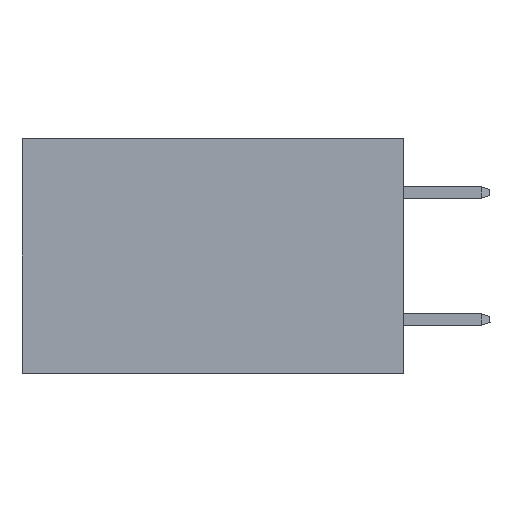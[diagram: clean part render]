
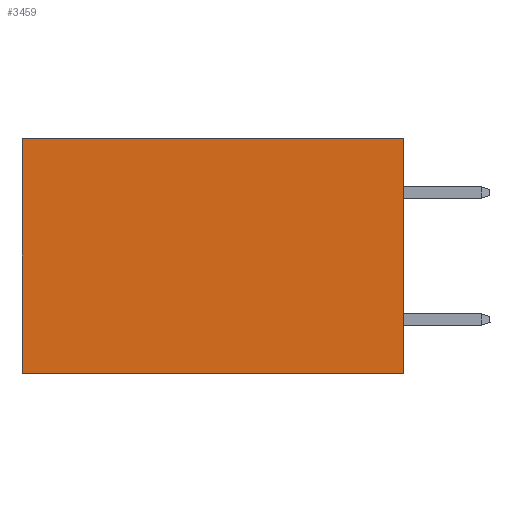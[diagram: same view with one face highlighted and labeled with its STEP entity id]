
A CAD part, left-side view. The second image highlights one B-rep face of the part: STEP entity #3459.
In plain terms, the highlighted planar face has unit normal (-1, 0, 0).
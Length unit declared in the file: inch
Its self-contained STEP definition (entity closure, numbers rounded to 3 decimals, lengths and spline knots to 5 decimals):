
#1199 = VERTEX_POINT ( 'NONE', #18235 ) ;
#1871 = DIRECTION ( 'NONE',  ( 0., 0., -1. ) ) ;
#3299 = DIRECTION ( 'NONE',  ( 1., 0., 0. ) ) ;
#3459 = ADVANCED_FACE ( 'NONE', ( #24115 ), #23495, .F. ) ;
#3513 = EDGE_LOOP ( 'NONE', ( #8835, #14694, #22181, #4053 ) ) ;
#3857 = LINE ( 'NONE', #20203, #14104 ) ;
#4053 = ORIENTED_EDGE ( 'NONE', *, *, #15301, .T. ) ;
#4644 = LINE ( 'NONE', #16486, #19744 ) ;
#7604 = EDGE_CURVE ( 'NONE', #12651, #15956, #9965, .T. ) ;
#8835 = ORIENTED_EDGE ( 'NONE', *, *, #22392, .T. ) ;
#8850 = VERTEX_POINT ( 'NONE', #9810 ) ;
#9133 = CARTESIAN_POINT ( 'NONE',  ( 0.2875, 0., -0.37 ) ) ;
#9810 = CARTESIAN_POINT ( 'NONE',  ( 0.2875, 0.6, 0. ) ) ;
#9911 = VECTOR ( 'NONE', #15269, 39.37008 ) ;
#9965 = LINE ( 'NONE', #24205, #11284 ) ;
#10450 = CARTESIAN_POINT ( 'NONE',  ( 0.2875, 0., 0. ) ) ;
#11261 = CARTESIAN_POINT ( 'NONE',  ( 0.2875, 0., 0. ) ) ;
#11284 = VECTOR ( 'NONE', #1871, 39.37008 ) ;
#11835 = DIRECTION ( 'NONE',  ( 0., 0., -1. ) ) ;
#12022 = CARTESIAN_POINT ( 'NONE',  ( 0.2875, 0., -0.37 ) ) ;
#12297 = EDGE_CURVE ( 'NONE', #15956, #1199, #25379, .T. ) ;
#12651 = VERTEX_POINT ( 'NONE', #10450 ) ;
#14104 = VECTOR ( 'NONE', #11835, 39.37008 ) ;
#14694 = ORIENTED_EDGE ( 'NONE', *, *, #12297, .F. ) ;
#15269 = DIRECTION ( 'NONE',  ( 0., 1., 0. ) ) ;
#15301 = EDGE_CURVE ( 'NONE', #12651, #8850, #4644, .T. ) ;
#15956 = VERTEX_POINT ( 'NONE', #12022 ) ;
#15983 = AXIS2_PLACEMENT_3D ( 'NONE', #11261, #3299, #25631 ) ;
#16486 = CARTESIAN_POINT ( 'NONE',  ( 0.2875, 0., 0. ) ) ;
#18235 = CARTESIAN_POINT ( 'NONE',  ( 0.2875, 0.6, -0.37 ) ) ;
#19744 = VECTOR ( 'NONE', #22452, 39.37008 ) ;
#20203 = CARTESIAN_POINT ( 'NONE',  ( 0.2875, 0.6, 0. ) ) ;
#22181 = ORIENTED_EDGE ( 'NONE', *, *, #7604, .F. ) ;
#22392 = EDGE_CURVE ( 'NONE', #8850, #1199, #3857, .T. ) ;
#22452 = DIRECTION ( 'NONE',  ( 0., 1., 0. ) ) ;
#23495 = PLANE ( 'NONE',  #15983 ) ;
#24115 = FACE_OUTER_BOUND ( 'NONE', #3513, .T. ) ;
#24205 = CARTESIAN_POINT ( 'NONE',  ( 0.2875, 0., 0. ) ) ;
#25379 = LINE ( 'NONE', #9133, #9911 ) ;
#25631 = DIRECTION ( 'NONE',  ( 0., 0., -1. ) ) ;
